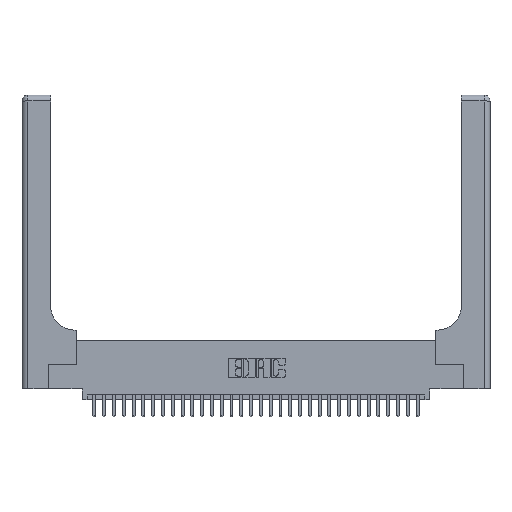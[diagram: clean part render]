
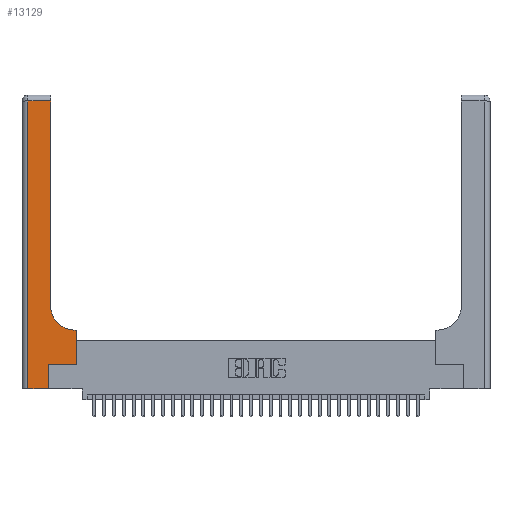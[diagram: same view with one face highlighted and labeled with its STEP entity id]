
A CAD part, top view. The second image highlights one B-rep face of the part: STEP entity #13129.
In plain terms, the highlighted planar face has unit normal (0, 0, 1).
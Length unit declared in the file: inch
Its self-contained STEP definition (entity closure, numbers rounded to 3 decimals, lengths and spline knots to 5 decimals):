
#331 = CARTESIAN_POINT ( 'NONE',  ( 0.5585, 0.25, 0.37 ) ) ;
#459 = CARTESIAN_POINT ( 'NONE',  ( 0., 3., 0.37 ) ) ;
#492 = VECTOR ( 'NONE', #4529, 39.37008 ) ;
#788 = LINE ( 'NONE', #16126, #30904 ) ;
#2184 = VERTEX_POINT ( 'NONE', #331 ) ;
#3068 = DIRECTION ( 'NONE',  ( -1., 0., 0. ) ) ;
#3115 = DIRECTION ( 'NONE',  ( 1., 0., 0. ) ) ;
#3174 = CARTESIAN_POINT ( 'NONE',  ( 0., 2.94, 0.37 ) ) ;
#3865 = LINE ( 'NONE', #15225, #32731 ) ;
#4529 = DIRECTION ( 'NONE',  ( 0., -1., 0. ) ) ;
#4619 = AXIS2_PLACEMENT_3D ( 'NONE', #459, #10947, #3068 ) ;
#5765 = DIRECTION ( 'NONE',  ( 0., 0., -1. ) ) ;
#6356 = EDGE_LOOP ( 'NONE', ( #17835, #26631, #12638, #15327, #16050, #32789, #16396, #9815, #14211 ) ) ;
#7514 = AXIS2_PLACEMENT_3D ( 'NONE', #23544, #5765, #18183 ) ;
#7561 = DIRECTION ( 'NONE',  ( 0., 1., 0. ) ) ;
#7776 = EDGE_CURVE ( 'NONE', #32968, #18715, #11127, .T. ) ;
#9296 = LINE ( 'NONE', #19062, #18441 ) ;
#9815 = ORIENTED_EDGE ( 'NONE', *, *, #14565, .T. ) ;
#9854 = LINE ( 'NONE', #29745, #492 ) ;
#10947 = DIRECTION ( 'NONE',  ( 0., 0., -1. ) ) ;
#11127 = CIRCLE ( 'NONE', #7514, 0.25 ) ;
#11443 = CARTESIAN_POINT ( 'NONE',  ( 0.269, 0.25, 0.37 ) ) ;
#11856 = CARTESIAN_POINT ( 'NONE',  ( 0.06, 0., 0.37 ) ) ;
#12638 = ORIENTED_EDGE ( 'NONE', *, *, #25294, .T. ) ;
#13129 = ADVANCED_FACE ( 'NONE', ( #14819 ), #26393, .F. ) ;
#14188 = VERTEX_POINT ( 'NONE', #15104 ) ;
#14211 = ORIENTED_EDGE ( 'NONE', *, *, #7776, .T. ) ;
#14565 = EDGE_CURVE ( 'NONE', #23507, #32968, #9296, .T. ) ;
#14787 = EDGE_CURVE ( 'NONE', #18715, #14188, #32460, .T. ) ;
#14819 = FACE_OUTER_BOUND ( 'NONE', #6356, .T. ) ;
#15104 = CARTESIAN_POINT ( 'NONE',  ( 0.2915, 2.94, 0.37 ) ) ;
#15225 = CARTESIAN_POINT ( 'NONE',  ( 0.269, 0., 0.37 ) ) ;
#15327 = ORIENTED_EDGE ( 'NONE', *, *, #32777, .T. ) ;
#15916 = CARTESIAN_POINT ( 'NONE',  ( 0.06, 2.94, 0.37 ) ) ;
#16050 = ORIENTED_EDGE ( 'NONE', *, *, #16817, .T. ) ;
#16126 = CARTESIAN_POINT ( 'NONE',  ( 0., 0., 0.37 ) ) ;
#16396 = ORIENTED_EDGE ( 'NONE', *, *, #18256, .T. ) ;
#16807 = DIRECTION ( 'NONE',  ( 0., 1., 0. ) ) ;
#16817 = EDGE_CURVE ( 'NONE', #28098, #18565, #3865, .T. ) ;
#17014 = CARTESIAN_POINT ( 'NONE',  ( 0.269, 0., 0.37 ) ) ;
#17132 = LINE ( 'NONE', #3174, #23915 ) ;
#17332 = DIRECTION ( 'NONE',  ( 0., 1., 0. ) ) ;
#17835 = ORIENTED_EDGE ( 'NONE', *, *, #14787, .T. ) ;
#18183 = DIRECTION ( 'NONE',  ( 1., 0., 0. ) ) ;
#18256 = EDGE_CURVE ( 'NONE', #2184, #23507, #29863, .T. ) ;
#18440 = CARTESIAN_POINT ( 'NONE',  ( 0.269, 0.25, 0.37 ) ) ;
#18441 = VECTOR ( 'NONE', #24215, 39.37008 ) ;
#18565 = VERTEX_POINT ( 'NONE', #11443 ) ;
#18685 = DIRECTION ( 'NONE',  ( 1., 0., 0. ) ) ;
#18715 = VERTEX_POINT ( 'NONE', #24535 ) ;
#19062 = CARTESIAN_POINT ( 'NONE',  ( 0.2915, 0.6, 0.37 ) ) ;
#19486 = CARTESIAN_POINT ( 'NONE',  ( 0.2915, 3., 0.37 ) ) ;
#19735 = CARTESIAN_POINT ( 'NONE',  ( 0.5585, 0.6, 0.37 ) ) ;
#20273 = VERTEX_POINT ( 'NONE', #11856 ) ;
#23079 = EDGE_CURVE ( 'NONE', #14188, #32741, #17132, .T. ) ;
#23507 = VERTEX_POINT ( 'NONE', #19735 ) ;
#23544 = CARTESIAN_POINT ( 'NONE',  ( 0.5415, 0.85, 0.37 ) ) ;
#23915 = VECTOR ( 'NONE', #26718, 39.37008 ) ;
#24215 = DIRECTION ( 'NONE',  ( -1., 0., 0. ) ) ;
#24535 = CARTESIAN_POINT ( 'NONE',  ( 0.2915, 0.85, 0.37 ) ) ;
#25294 = EDGE_CURVE ( 'NONE', #32741, #20273, #9854, .T. ) ;
#25457 = VECTOR ( 'NONE', #7561, 39.37008 ) ;
#26393 = PLANE ( 'NONE',  #4619 ) ;
#26631 = ORIENTED_EDGE ( 'NONE', *, *, #23079, .T. ) ;
#26718 = DIRECTION ( 'NONE',  ( -1., 0., 0. ) ) ;
#26770 = VECTOR ( 'NONE', #3115, 39.37008 ) ;
#27797 = EDGE_CURVE ( 'NONE', #18565, #2184, #28408, .T. ) ;
#28098 = VERTEX_POINT ( 'NONE', #17014 ) ;
#28408 = LINE ( 'NONE', #18440, #26770 ) ;
#29745 = CARTESIAN_POINT ( 'NONE',  ( 0.06, 3., 0.37 ) ) ;
#29863 = LINE ( 'NONE', #30840, #25457 ) ;
#30840 = CARTESIAN_POINT ( 'NONE',  ( 0.5585, 0.25, 0.37 ) ) ;
#30904 = VECTOR ( 'NONE', #18685, 39.37008 ) ;
#31584 = CARTESIAN_POINT ( 'NONE',  ( 0.5415, 0.6, 0.37 ) ) ;
#32460 = LINE ( 'NONE', #19486, #32892 ) ;
#32731 = VECTOR ( 'NONE', #17332, 39.37008 ) ;
#32741 = VERTEX_POINT ( 'NONE', #15916 ) ;
#32777 = EDGE_CURVE ( 'NONE', #20273, #28098, #788, .T. ) ;
#32789 = ORIENTED_EDGE ( 'NONE', *, *, #27797, .T. ) ;
#32892 = VECTOR ( 'NONE', #16807, 39.37008 ) ;
#32968 = VERTEX_POINT ( 'NONE', #31584 ) ;
